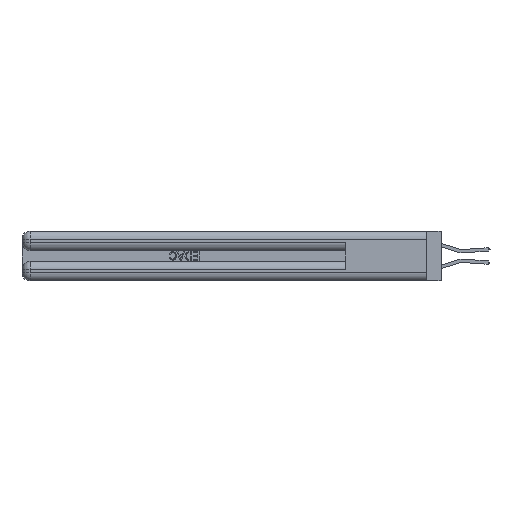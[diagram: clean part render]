
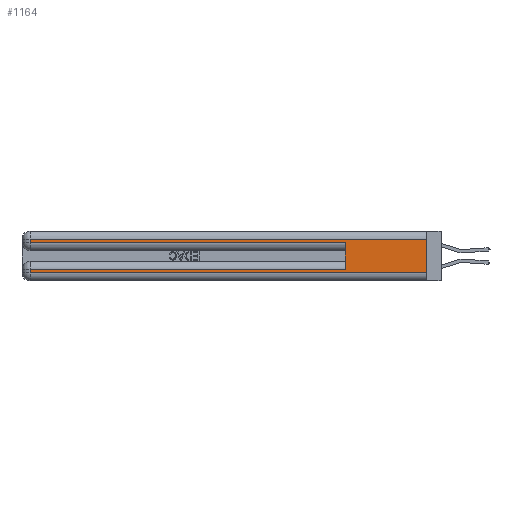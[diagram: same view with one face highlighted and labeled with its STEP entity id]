
A CAD part, left-side view. The second image highlights one B-rep face of the part: STEP entity #1164.
In plain terms, the highlighted planar face has unit normal (-1, 0, 0).
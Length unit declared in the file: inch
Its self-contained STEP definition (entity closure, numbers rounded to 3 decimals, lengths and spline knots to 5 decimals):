
#675 = VECTOR ( 'NONE', #32793, 39.37008 ) ;
#692 = EDGE_CURVE ( 'NONE', #4497, #38605, #14170, .T. ) ;
#1164 = ADVANCED_FACE ( 'NONE', ( #3788 ), #32856, .F. ) ;
#1767 = EDGE_CURVE ( 'NONE', #35718, #4337, #27315, .T. ) ;
#2364 = DIRECTION ( 'NONE',  ( 0., 1., 0. ) ) ;
#2903 = ORIENTED_EDGE ( 'NONE', *, *, #1767, .T. ) ;
#3052 = LINE ( 'NONE', #11350, #33295 ) ;
#3788 = FACE_OUTER_BOUND ( 'NONE', #24580, .T. ) ;
#4270 = DIRECTION ( 'NONE',  ( 0., 0., 1. ) ) ;
#4337 = VERTEX_POINT ( 'NONE', #31769 ) ;
#4497 = VERTEX_POINT ( 'NONE', #35487 ) ;
#5309 = LINE ( 'NONE', #7984, #35441 ) ;
#7124 = CARTESIAN_POINT ( 'NONE',  ( 0., 2.94, 0.06 ) ) ;
#7870 = ORIENTED_EDGE ( 'NONE', *, *, #13780, .T. ) ;
#7984 = CARTESIAN_POINT ( 'NONE',  ( 0., 0., 0.37 ) ) ;
#8124 = DIRECTION ( 'NONE',  ( 0., 1., 0. ) ) ;
#9013 = EDGE_CURVE ( 'NONE', #34623, #4337, #5309, .T. ) ;
#11350 = CARTESIAN_POINT ( 'NONE',  ( 0., 0.6, 0.145 ) ) ;
#12099 = ORIENTED_EDGE ( 'NONE', *, *, #12447, .T. ) ;
#12447 = EDGE_CURVE ( 'NONE', #34623, #35804, #30603, .T. ) ;
#13780 = EDGE_CURVE ( 'NONE', #35804, #4497, #33266, .T. ) ;
#14170 = LINE ( 'NONE', #14171, #23185 ) ;
#14171 = CARTESIAN_POINT ( 'NONE',  ( 0., 0., 0.285 ) ) ;
#15005 = CARTESIAN_POINT ( 'NONE',  ( 0., 0., 0.31 ) ) ;
#15540 = CARTESIAN_POINT ( 'NONE',  ( 0., 0.6, 0.285 ) ) ;
#16145 = AXIS2_PLACEMENT_3D ( 'NONE', #20920, #35818, #18022 ) ;
#17048 = CARTESIAN_POINT ( 'NONE',  ( 0., 2.94, 0.31 ) ) ;
#17255 = DIRECTION ( 'NONE',  ( 0., -1., 0. ) ) ;
#17555 = CARTESIAN_POINT ( 'NONE',  ( 0., 0., 0.085 ) ) ;
#17995 = LINE ( 'NONE', #29825, #675 ) ;
#18022 = DIRECTION ( 'NONE',  ( 0., 0., -1. ) ) ;
#19072 = ORIENTED_EDGE ( 'NONE', *, *, #30876, .T. ) ;
#20261 = DIRECTION ( 'NONE',  ( 0., -1., 0. ) ) ;
#20300 = CARTESIAN_POINT ( 'NONE',  ( 0., 0., 0.31 ) ) ;
#20920 = CARTESIAN_POINT ( 'NONE',  ( 0., 0., 0.37 ) ) ;
#21114 = ORIENTED_EDGE ( 'NONE', *, *, #692, .T. ) ;
#21657 = ORIENTED_EDGE ( 'NONE', *, *, #30924, .T. ) ;
#21848 = VERTEX_POINT ( 'NONE', #36814 ) ;
#23185 = VECTOR ( 'NONE', #17255, 39.37008 ) ;
#24580 = EDGE_LOOP ( 'NONE', ( #32965, #12099, #7870, #21114, #37987, #19072, #21657, #2903 ) ) ;
#25450 = VECTOR ( 'NONE', #20261, 39.37008 ) ;
#25999 = VECTOR ( 'NONE', #2364, 39.37008 ) ;
#26212 = DIRECTION ( 'NONE',  ( 0., 0., -1. ) ) ;
#26921 = LINE ( 'NONE', #17555, #25999 ) ;
#27315 = LINE ( 'NONE', #35025, #25450 ) ;
#28405 = CARTESIAN_POINT ( 'NONE',  ( 0., 0.6, 0.085 ) ) ;
#28843 = EDGE_CURVE ( 'NONE', #34386, #38605, #3052, .T. ) ;
#29825 = CARTESIAN_POINT ( 'NONE',  ( 0., 2.94, 0.37 ) ) ;
#30603 = LINE ( 'NONE', #20300, #37523 ) ;
#30876 = EDGE_CURVE ( 'NONE', #34386, #21848, #26921, .T. ) ;
#30924 = EDGE_CURVE ( 'NONE', #21848, #35718, #17995, .T. ) ;
#31769 = CARTESIAN_POINT ( 'NONE',  ( 0., 0., 0.06 ) ) ;
#32169 = CARTESIAN_POINT ( 'NONE',  ( 0., 2.94, 0.37 ) ) ;
#32356 = VECTOR ( 'NONE', #35107, 39.37008 ) ;
#32793 = DIRECTION ( 'NONE',  ( 0., 0., -1. ) ) ;
#32856 = PLANE ( 'NONE',  #16145 ) ;
#32965 = ORIENTED_EDGE ( 'NONE', *, *, #9013, .F. ) ;
#33266 = LINE ( 'NONE', #32169, #32356 ) ;
#33295 = VECTOR ( 'NONE', #4270, 39.37008 ) ;
#34386 = VERTEX_POINT ( 'NONE', #28405 ) ;
#34623 = VERTEX_POINT ( 'NONE', #15005 ) ;
#35025 = CARTESIAN_POINT ( 'NONE',  ( 0., 0., 0.06 ) ) ;
#35107 = DIRECTION ( 'NONE',  ( 0., 0., -1. ) ) ;
#35441 = VECTOR ( 'NONE', #26212, 39.37008 ) ;
#35487 = CARTESIAN_POINT ( 'NONE',  ( 0., 2.94, 0.285 ) ) ;
#35718 = VERTEX_POINT ( 'NONE', #7124 ) ;
#35804 = VERTEX_POINT ( 'NONE', #17048 ) ;
#35818 = DIRECTION ( 'NONE',  ( 1., 0., 0. ) ) ;
#36814 = CARTESIAN_POINT ( 'NONE',  ( 0., 2.94, 0.085 ) ) ;
#37523 = VECTOR ( 'NONE', #8124, 39.37008 ) ;
#37987 = ORIENTED_EDGE ( 'NONE', *, *, #28843, .F. ) ;
#38605 = VERTEX_POINT ( 'NONE', #15540 ) ;
